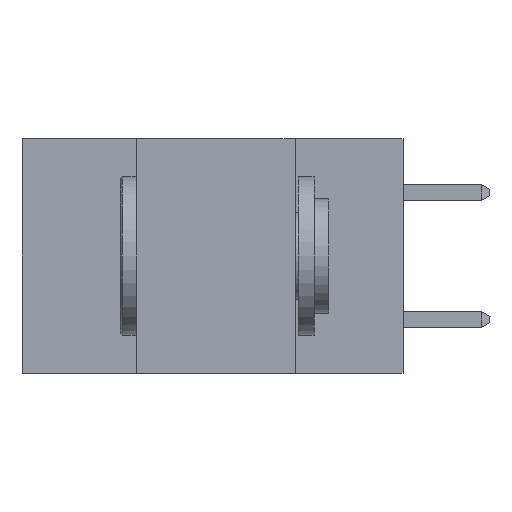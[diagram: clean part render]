
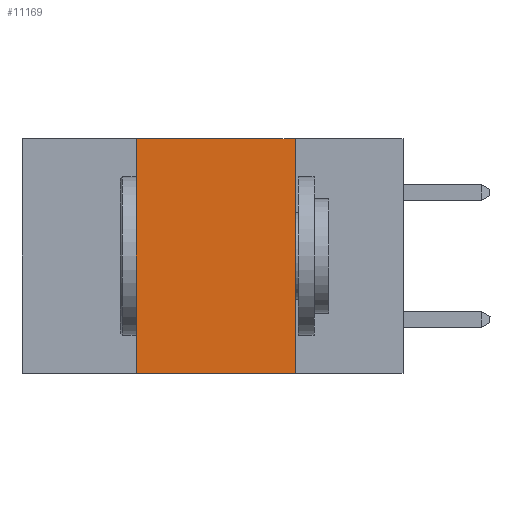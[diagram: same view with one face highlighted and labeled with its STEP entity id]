
A CAD part, left-side view. The second image highlights one B-rep face of the part: STEP entity #11169.
In plain terms, the highlighted planar face has unit normal (-1, 0, 0).
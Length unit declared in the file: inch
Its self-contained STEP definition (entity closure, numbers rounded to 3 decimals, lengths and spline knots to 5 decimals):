
#519 = VERTEX_POINT ( 'NONE', #17613 ) ;
#1105 = DIRECTION ( 'NONE',  ( 0., 0., -1. ) ) ;
#1752 = VECTOR ( 'NONE', #10793, 39.37008 ) ;
#1847 = EDGE_CURVE ( 'NONE', #11997, #519, #18530, .T. ) ;
#2195 = EDGE_CURVE ( 'NONE', #11997, #19955, #19957, .T. ) ;
#2645 = ORIENTED_EDGE ( 'NONE', *, *, #18446, .F. ) ;
#3237 = ORIENTED_EDGE ( 'NONE', *, *, #1847, .T. ) ;
#3341 = CARTESIAN_POINT ( 'NONE',  ( 0., 0.42, 0. ) ) ;
#3479 = CARTESIAN_POINT ( 'NONE',  ( 0., 0.17, 0. ) ) ;
#3563 = VECTOR ( 'NONE', #6829, 39.37008 ) ;
#4111 = CARTESIAN_POINT ( 'NONE',  ( 0., 0.42, -0.37 ) ) ;
#4677 = ORIENTED_EDGE ( 'NONE', *, *, #14257, .F. ) ;
#5906 = VECTOR ( 'NONE', #19580, 39.37008 ) ;
#6343 = VERTEX_POINT ( 'NONE', #3479 ) ;
#6829 = DIRECTION ( 'NONE',  ( 0., 0., -1. ) ) ;
#7162 = FACE_OUTER_BOUND ( 'NONE', #15747, .T. ) ;
#7775 = CARTESIAN_POINT ( 'NONE',  ( 0., 0.17, 0. ) ) ;
#8869 = AXIS2_PLACEMENT_3D ( 'NONE', #14991, #18011, #1105 ) ;
#9270 = CARTESIAN_POINT ( 'NONE',  ( 0., 0.6, 0. ) ) ;
#10793 = DIRECTION ( 'NONE',  ( 0., -1., 0. ) ) ;
#10962 = DIRECTION ( 'NONE',  ( 0., 0., 1. ) ) ;
#11169 = ADVANCED_FACE ( 'NONE', ( #7162 ), #11639, .F. ) ;
#11639 = PLANE ( 'NONE',  #8869 ) ;
#11997 = VERTEX_POINT ( 'NONE', #4111 ) ;
#13310 = CARTESIAN_POINT ( 'NONE',  ( 0., 0.6, -0.37 ) ) ;
#14257 = EDGE_CURVE ( 'NONE', #19955, #6343, #17792, .T. ) ;
#14456 = LINE ( 'NONE', #7775, #3563 ) ;
#14991 = CARTESIAN_POINT ( 'NONE',  ( 0., 0.6, 0. ) ) ;
#15578 = VECTOR ( 'NONE', #10962, 39.37008 ) ;
#15747 = EDGE_LOOP ( 'NONE', ( #2645, #4677, #19807, #3237 ) ) ;
#16195 = CARTESIAN_POINT ( 'NONE',  ( 0., 0.42, 0. ) ) ;
#17613 = CARTESIAN_POINT ( 'NONE',  ( 0., 0.17, -0.37 ) ) ;
#17792 = LINE ( 'NONE', #9270, #1752 ) ;
#18011 = DIRECTION ( 'NONE',  ( 1., 0., 0. ) ) ;
#18446 = EDGE_CURVE ( 'NONE', #6343, #519, #14456, .T. ) ;
#18530 = LINE ( 'NONE', #13310, #5906 ) ;
#19580 = DIRECTION ( 'NONE',  ( 0., -1., 0. ) ) ;
#19807 = ORIENTED_EDGE ( 'NONE', *, *, #2195, .F. ) ;
#19955 = VERTEX_POINT ( 'NONE', #16195 ) ;
#19957 = LINE ( 'NONE', #3341, #15578 ) ;
